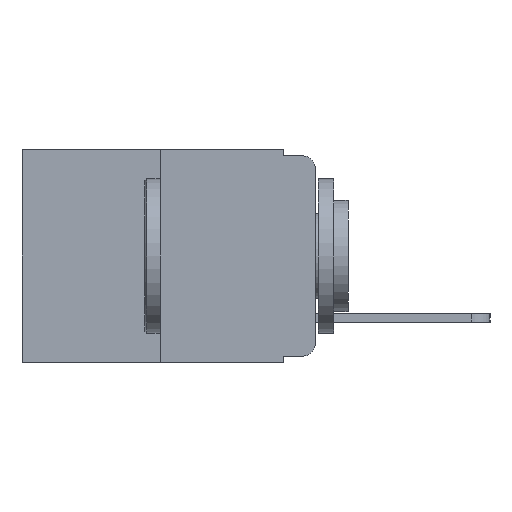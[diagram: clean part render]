
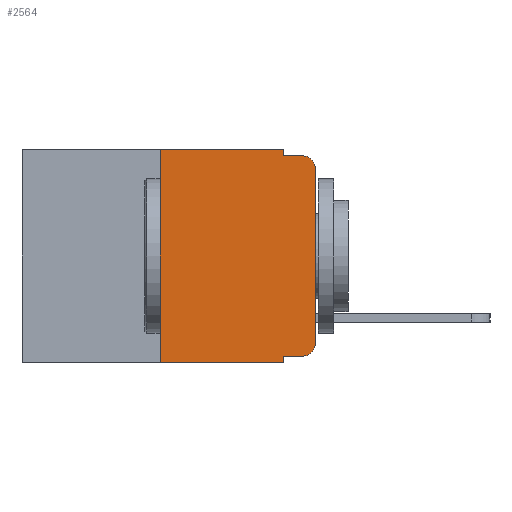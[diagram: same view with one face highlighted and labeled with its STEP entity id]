
A CAD part, left-side view. The second image highlights one B-rep face of the part: STEP entity #2564.
In plain terms, the highlighted planar face has unit normal (-1, 0, 0).
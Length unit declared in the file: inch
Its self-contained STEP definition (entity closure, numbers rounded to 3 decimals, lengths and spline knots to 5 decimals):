
#72 = ORIENTED_EDGE ( 'NONE', *, *, #910, .F. ) ;
#145 = ORIENTED_EDGE ( 'NONE', *, *, #17879, .F. ) ;
#725 = CARTESIAN_POINT ( 'NONE',  ( 0., 0.473, 0. ) ) ;
#910 = EDGE_CURVE ( 'NONE', #16777, #3469, #14751, .T. ) ;
#1117 = ORIENTED_EDGE ( 'NONE', *, *, #16861, .F. ) ;
#1326 = ORIENTED_EDGE ( 'NONE', *, *, #1939, .F. ) ;
#1489 = CARTESIAN_POINT ( 'NONE',  ( 0., 0.25, -0.343 ) ) ;
#1702 = DIRECTION ( 'NONE',  ( 0., -1., 0. ) ) ;
#1939 = EDGE_CURVE ( 'NONE', #3469, #16320, #11317, .T. ) ;
#2261 = EDGE_LOOP ( 'NONE', ( #11683, #14966, #1326, #72, #9915, #145, #8631, #1117, #9961, #3576 ) ) ;
#2564 = ADVANCED_FACE ( 'NONE', ( #16076 ), #16510, .F. ) ;
#2981 = AXIS2_PLACEMENT_3D ( 'NONE', #725, #5674, #3941 ) ;
#2990 = CARTESIAN_POINT ( 'NONE',  ( 0., 0.25, 0. ) ) ;
#3469 = VERTEX_POINT ( 'NONE', #16327 ) ;
#3576 = ORIENTED_EDGE ( 'NONE', *, *, #12791, .T. ) ;
#3941 = DIRECTION ( 'NONE',  ( 0., 0., -1. ) ) ;
#4516 = CARTESIAN_POINT ( 'NONE',  ( 0., 0.02, -0.03 ) ) ;
#4609 = CARTESIAN_POINT ( 'NONE',  ( 0., 0.051, 0. ) ) ;
#4837 = CARTESIAN_POINT ( 'NONE',  ( 0., 0.02, -0.313 ) ) ;
#5331 = VECTOR ( 'NONE', #10648, 39.37008 ) ;
#5674 = DIRECTION ( 'NONE',  ( 1., 0., 0. ) ) ;
#5995 = VERTEX_POINT ( 'NONE', #18663 ) ;
#6119 = EDGE_CURVE ( 'NONE', #14514, #16320, #17460, .T. ) ;
#6415 = DIRECTION ( 'NONE',  ( 0., 0., -1. ) ) ;
#6433 = VECTOR ( 'NONE', #1702, 39.37008 ) ;
#6516 = CARTESIAN_POINT ( 'NONE',  ( 0., 0.051, 0. ) ) ;
#6718 = VERTEX_POINT ( 'NONE', #1489 ) ;
#6786 = LINE ( 'NONE', #15753, #16884 ) ;
#6997 = CARTESIAN_POINT ( 'NONE',  ( 0., 0., -0.03 ) ) ;
#7339 = CARTESIAN_POINT ( 'NONE',  ( 0., 0.051, -0.333 ) ) ;
#7430 = VERTEX_POINT ( 'NONE', #7339 ) ;
#7518 = CIRCLE ( 'NONE', #16489, 0.02 ) ;
#8631 = ORIENTED_EDGE ( 'NONE', *, *, #17761, .T. ) ;
#8724 = LINE ( 'NONE', #16644, #16449 ) ;
#9065 = CARTESIAN_POINT ( 'NONE',  ( 0., 0.051, -0.333 ) ) ;
#9273 = EDGE_CURVE ( 'NONE', #16316, #14514, #9668, .T. ) ;
#9668 = LINE ( 'NONE', #18208, #13311 ) ;
#9712 = CARTESIAN_POINT ( 'NONE',  ( 0., 0., -0.313 ) ) ;
#9915 = ORIENTED_EDGE ( 'NONE', *, *, #10095, .F. ) ;
#9961 = ORIENTED_EDGE ( 'NONE', *, *, #15854, .T. ) ;
#10095 = EDGE_CURVE ( 'NONE', #17861, #16777, #10129, .T. ) ;
#10129 = LINE ( 'NONE', #12613, #6433 ) ;
#10463 = LINE ( 'NONE', #15475, #18081 ) ;
#10648 = DIRECTION ( 'NONE',  ( 0., -1., 0. ) ) ;
#11136 = DIRECTION ( 'NONE',  ( 0., 0., -1. ) ) ;
#11317 = LINE ( 'NONE', #12981, #11793 ) ;
#11683 = ORIENTED_EDGE ( 'NONE', *, *, #9273, .T. ) ;
#11793 = VECTOR ( 'NONE', #12860, 39.37008 ) ;
#11897 = DIRECTION ( 'NONE',  ( 0., 0., -1. ) ) ;
#12613 = CARTESIAN_POINT ( 'NONE',  ( 0., 0.473, 0. ) ) ;
#12791 = EDGE_CURVE ( 'NONE', #5995, #16316, #7518, .T. ) ;
#12860 = DIRECTION ( 'NONE',  ( 0., -1., 0. ) ) ;
#12864 = VERTEX_POINT ( 'NONE', #18831 ) ;
#12981 = CARTESIAN_POINT ( 'NONE',  ( 0., 0.051, -0.01 ) ) ;
#13311 = VECTOR ( 'NONE', #19703, 39.37008 ) ;
#14411 = AXIS2_PLACEMENT_3D ( 'NONE', #4516, #14543, #17940 ) ;
#14514 = VERTEX_POINT ( 'NONE', #6997 ) ;
#14543 = DIRECTION ( 'NONE',  ( -1., 0., 0. ) ) ;
#14751 = LINE ( 'NONE', #6516, #18708 ) ;
#14966 = ORIENTED_EDGE ( 'NONE', *, *, #6119, .T. ) ;
#15475 = CARTESIAN_POINT ( 'NONE',  ( 0., 0.25, 0. ) ) ;
#15708 = DIRECTION ( 'NONE',  ( -1., 0., 0. ) ) ;
#15753 = CARTESIAN_POINT ( 'NONE',  ( 0., 0.051, 0. ) ) ;
#15854 = EDGE_CURVE ( 'NONE', #7430, #5995, #17179, .T. ) ;
#15899 = CARTESIAN_POINT ( 'NONE',  ( 0., 0.02, -0.01 ) ) ;
#16076 = FACE_OUTER_BOUND ( 'NONE', #2261, .T. ) ;
#16316 = VERTEX_POINT ( 'NONE', #9712 ) ;
#16320 = VERTEX_POINT ( 'NONE', #15899 ) ;
#16327 = CARTESIAN_POINT ( 'NONE',  ( 0., 0.051, -0.01 ) ) ;
#16449 = VECTOR ( 'NONE', #19641, 39.37008 ) ;
#16489 = AXIS2_PLACEMENT_3D ( 'NONE', #4837, #15708, #6415 ) ;
#16510 = PLANE ( 'NONE',  #2981 ) ;
#16644 = CARTESIAN_POINT ( 'NONE',  ( 0., 0.473, -0.343 ) ) ;
#16777 = VERTEX_POINT ( 'NONE', #4609 ) ;
#16861 = EDGE_CURVE ( 'NONE', #7430, #12864, #6786, .T. ) ;
#16884 = VECTOR ( 'NONE', #11136, 39.37008 ) ;
#16961 = DIRECTION ( 'NONE',  ( 0., 0., 1. ) ) ;
#17179 = LINE ( 'NONE', #9065, #5331 ) ;
#17460 = CIRCLE ( 'NONE', #14411, 0.02 ) ;
#17761 = EDGE_CURVE ( 'NONE', #6718, #12864, #8724, .T. ) ;
#17861 = VERTEX_POINT ( 'NONE', #2990 ) ;
#17879 = EDGE_CURVE ( 'NONE', #6718, #17861, #10463, .T. ) ;
#17940 = DIRECTION ( 'NONE',  ( 0., 0., -1. ) ) ;
#18081 = VECTOR ( 'NONE', #16961, 39.37008 ) ;
#18208 = CARTESIAN_POINT ( 'NONE',  ( 0., 0., 0. ) ) ;
#18663 = CARTESIAN_POINT ( 'NONE',  ( 0., 0.02, -0.333 ) ) ;
#18708 = VECTOR ( 'NONE', #11897, 39.37008 ) ;
#18831 = CARTESIAN_POINT ( 'NONE',  ( 0., 0.051, -0.343 ) ) ;
#19641 = DIRECTION ( 'NONE',  ( 0., -1., 0. ) ) ;
#19703 = DIRECTION ( 'NONE',  ( 0., 0., 1. ) ) ;
